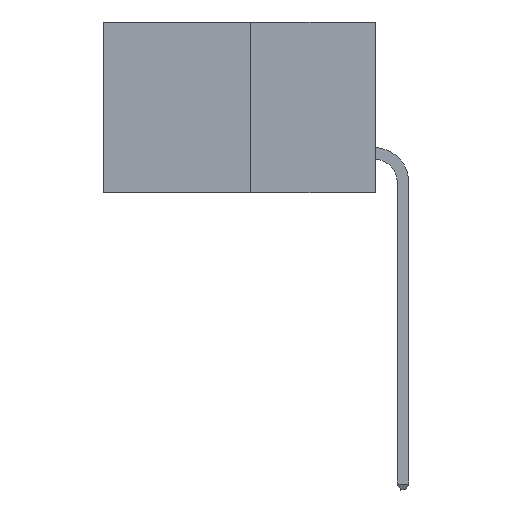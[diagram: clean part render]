
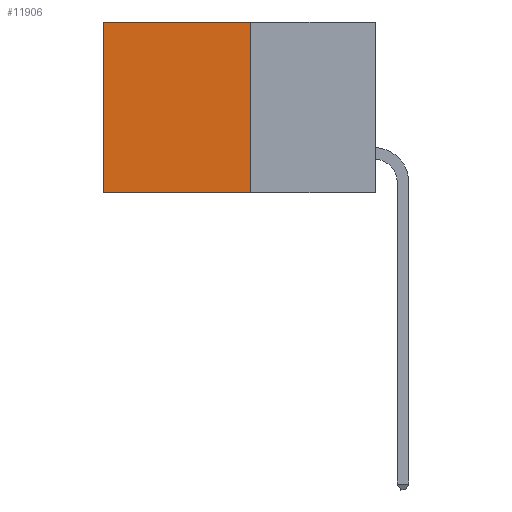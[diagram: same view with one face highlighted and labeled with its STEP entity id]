
A CAD part, left-side view. The second image highlights one B-rep face of the part: STEP entity #11906.
In plain terms, the highlighted planar face has unit normal (-1, 0, 0).
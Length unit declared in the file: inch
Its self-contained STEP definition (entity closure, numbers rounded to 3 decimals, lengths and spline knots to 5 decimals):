
#4 = DIRECTION ( 'NONE',  ( 0., 1., 0. ) ) ;
#104 = CARTESIAN_POINT ( 'NONE',  ( 0.277, 0.27, 0. ) ) ;
#231 = CARTESIAN_POINT ( 'NONE',  ( 0.277, 0.27, -0.37 ) ) ;
#671 = VERTEX_POINT ( 'NONE', #6021 ) ;
#765 = CARTESIAN_POINT ( 'NONE',  ( 0.277, 0.27, 0. ) ) ;
#1167 = ORIENTED_EDGE ( 'NONE', *, *, #2136, .T. ) ;
#1207 = LINE ( 'NONE', #4304, #1862 ) ;
#1862 = VECTOR ( 'NONE', #12449, 39.37008 ) ;
#2136 = EDGE_CURVE ( 'NONE', #9888, #3271, #11029, .T. ) ;
#2413 = EDGE_LOOP ( 'NONE', ( #3240, #11424, #9050, #1167 ) ) ;
#2486 = AXIS2_PLACEMENT_3D ( 'NONE', #11148, #12161, #6100 ) ;
#2922 = CARTESIAN_POINT ( 'NONE',  ( 0.277, 0.27, -0.37 ) ) ;
#3148 = VECTOR ( 'NONE', #4, 39.37008 ) ;
#3240 = ORIENTED_EDGE ( 'NONE', *, *, #6411, .T. ) ;
#3271 = VERTEX_POINT ( 'NONE', #12217 ) ;
#3770 = VERTEX_POINT ( 'NONE', #231 ) ;
#3996 = PLANE ( 'NONE',  #2486 ) ;
#4304 = CARTESIAN_POINT ( 'NONE',  ( 0.277, 0.59, -0.37 ) ) ;
#4598 = LINE ( 'NONE', #2922, #7670 ) ;
#5505 = VECTOR ( 'NONE', #11611, 39.37008 ) ;
#5831 = LINE ( 'NONE', #6578, #5505 ) ;
#6021 = CARTESIAN_POINT ( 'NONE',  ( 0.277, 0.59, -0.37 ) ) ;
#6100 = DIRECTION ( 'NONE',  ( 0., 0., -1. ) ) ;
#6411 = EDGE_CURVE ( 'NONE', #3271, #671, #1207, .T. ) ;
#6578 = CARTESIAN_POINT ( 'NONE',  ( 0.277, 0.27, -0.37 ) ) ;
#7670 = VECTOR ( 'NONE', #10121, 39.37008 ) ;
#9050 = ORIENTED_EDGE ( 'NONE', *, *, #12560, .F. ) ;
#9321 = EDGE_CURVE ( 'NONE', #3770, #671, #5831, .T. ) ;
#9888 = VERTEX_POINT ( 'NONE', #765 ) ;
#10121 = DIRECTION ( 'NONE',  ( 0., 0., -1. ) ) ;
#11029 = LINE ( 'NONE', #104, #3148 ) ;
#11148 = CARTESIAN_POINT ( 'NONE',  ( 0.277, 0.27, -0.37 ) ) ;
#11424 = ORIENTED_EDGE ( 'NONE', *, *, #9321, .F. ) ;
#11611 = DIRECTION ( 'NONE',  ( 0., 1., 0. ) ) ;
#11906 = ADVANCED_FACE ( 'NONE', ( #12257 ), #3996, .F. ) ;
#12161 = DIRECTION ( 'NONE',  ( 1., 0., 0. ) ) ;
#12217 = CARTESIAN_POINT ( 'NONE',  ( 0.277, 0.59, 0. ) ) ;
#12257 = FACE_OUTER_BOUND ( 'NONE', #2413, .T. ) ;
#12449 = DIRECTION ( 'NONE',  ( 0., 0., -1. ) ) ;
#12560 = EDGE_CURVE ( 'NONE', #9888, #3770, #4598, .T. ) ;
